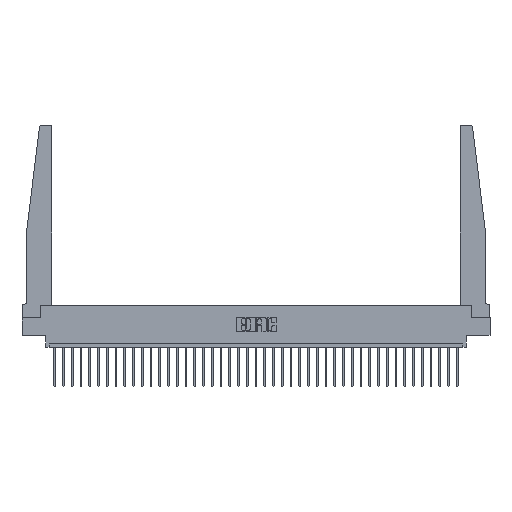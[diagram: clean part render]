
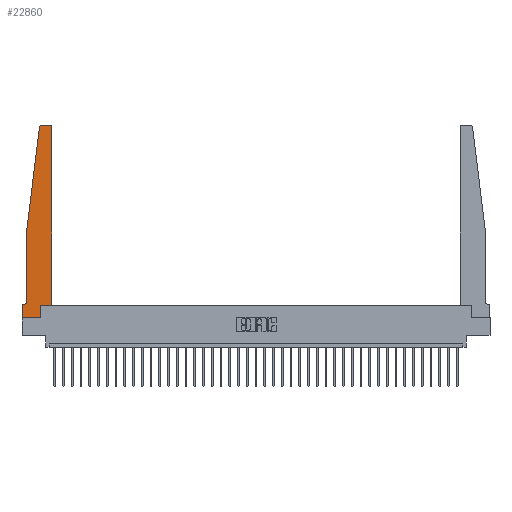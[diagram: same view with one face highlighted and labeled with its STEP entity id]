
A CAD part, top view. The second image highlights one B-rep face of the part: STEP entity #22860.
In plain terms, the highlighted planar face has unit normal (0, 0, 1).
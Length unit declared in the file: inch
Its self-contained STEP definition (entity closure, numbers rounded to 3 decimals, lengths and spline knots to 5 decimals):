
#249 = CARTESIAN_POINT ( 'NONE',  ( 0.065, 1.25, 0.37 ) ) ;
#384 = DIRECTION ( 'NONE',  ( 0., 1., 0. ) ) ;
#1217 = CIRCLE ( 'NONE', #8306, 0.03 ) ;
#1601 = CARTESIAN_POINT ( 'NONE',  ( 0.395, 2.75, 0.37 ) ) ;
#1854 = EDGE_CURVE ( 'NONE', #15519, #19445, #18045, .T. ) ;
#1911 = VECTOR ( 'NONE', #4742, 39.37008 ) ;
#2056 = AXIS2_PLACEMENT_3D ( 'NONE', #18401, #25612, #10159 ) ;
#2372 = CARTESIAN_POINT ( 'NONE',  ( 0.27653, 2.75, 0.37 ) ) ;
#3212 = LINE ( 'NONE', #31163, #17536 ) ;
#3720 = LINE ( 'NONE', #24644, #11105 ) ;
#3906 = VERTEX_POINT ( 'NONE', #32244 ) ;
#4670 = ORIENTED_EDGE ( 'NONE', *, *, #16605, .T. ) ;
#4693 = PLANE ( 'NONE',  #2056 ) ;
#4742 = DIRECTION ( 'NONE',  ( 1., 0., 0. ) ) ;
#4964 = CARTESIAN_POINT ( 'NONE',  ( 0.2605, 0.18, 0.37 ) ) ;
#5405 = ORIENTED_EDGE ( 'NONE', *, *, #1854, .T. ) ;
#6038 = EDGE_CURVE ( 'NONE', #16169, #17332, #11940, .T. ) ;
#6305 = EDGE_CURVE ( 'NONE', #3906, #33492, #29729, .T. ) ;
#7062 = CARTESIAN_POINT ( 'NONE',  ( 0., 0., 0.37 ) ) ;
#7340 = VECTOR ( 'NONE', #13923, 39.37008 ) ;
#7753 = CARTESIAN_POINT ( 'NONE',  ( 0., 0., 0.37 ) ) ;
#7915 = FACE_OUTER_BOUND ( 'NONE', #7938, .T. ) ;
#7938 = EDGE_LOOP ( 'NONE', ( #4670, #33658, #24033, #18374, #13474, #18819, #27400, #5405, #24749, #27364, #28347, #12217 ) ) ;
#8264 = DIRECTION ( 'NONE',  ( -1., 0., 0. ) ) ;
#8306 = AXIS2_PLACEMENT_3D ( 'NONE', #10468, #20936, #28463 ) ;
#8775 = LINE ( 'NONE', #10841, #7340 ) ;
#8815 = DIRECTION ( 'NONE',  ( 0., 0., 1. ) ) ;
#8956 = VECTOR ( 'NONE', #10697, 39.37008 ) ;
#9707 = LINE ( 'NONE', #25494, #1911 ) ;
#10068 = EDGE_CURVE ( 'NONE', #30839, #16169, #1217, .T. ) ;
#10159 = DIRECTION ( 'NONE',  ( 1., 0., 0. ) ) ;
#10468 = CARTESIAN_POINT ( 'NONE',  ( 0.27653, 2.72, 0.37 ) ) ;
#10549 = VECTOR ( 'NONE', #28042, 39.37008 ) ;
#10682 = LINE ( 'NONE', #18757, #19013 ) ;
#10697 = DIRECTION ( 'NONE',  ( -1., 0., 0. ) ) ;
#10841 = CARTESIAN_POINT ( 'NONE',  ( 0.2605, 0.18, 0.37 ) ) ;
#10946 = EDGE_CURVE ( 'NONE', #12994, #21836, #20360, .T. ) ;
#11105 = VECTOR ( 'NONE', #31818, 39.37008 ) ;
#11562 = CARTESIAN_POINT ( 'NONE',  ( 0.395, 2.72, 0.37 ) ) ;
#11940 = LINE ( 'NONE', #32853, #10549 ) ;
#12217 = ORIENTED_EDGE ( 'NONE', *, *, #6305, .T. ) ;
#12855 = CARTESIAN_POINT ( 'NONE',  ( 0.065, 0.2375, 0.37 ) ) ;
#12994 = VERTEX_POINT ( 'NONE', #12855 ) ;
#13065 = CARTESIAN_POINT ( 'NONE',  ( 0.425, 0.18, 0.37 ) ) ;
#13287 = AXIS2_PLACEMENT_3D ( 'NONE', #11562, #8815, #29732 ) ;
#13474 = ORIENTED_EDGE ( 'NONE', *, *, #10946, .T. ) ;
#13923 = DIRECTION ( 'NONE',  ( 0., 1., 0. ) ) ;
#15147 = EDGE_CURVE ( 'NONE', #21836, #23645, #17765, .T. ) ;
#15519 = VERTEX_POINT ( 'NONE', #7753 ) ;
#16169 = VERTEX_POINT ( 'NONE', #20392 ) ;
#16605 = EDGE_CURVE ( 'NONE', #33492, #30839, #3720, .T. ) ;
#16638 = CARTESIAN_POINT ( 'NONE',  ( 0.015, 0.1875, 0.37 ) ) ;
#17256 = EDGE_CURVE ( 'NONE', #19445, #19138, #8775, .T. ) ;
#17332 = VERTEX_POINT ( 'NONE', #249 ) ;
#17536 = VECTOR ( 'NONE', #18169, 39.37008 ) ;
#17765 = LINE ( 'NONE', #25645, #8956 ) ;
#17890 = EDGE_CURVE ( 'NONE', #19138, #26549, #9707, .T. ) ;
#17979 = CARTESIAN_POINT ( 'NONE',  ( 0.2605, 0., 0.37 ) ) ;
#18045 = LINE ( 'NONE', #7062, #32635 ) ;
#18169 = DIRECTION ( 'NONE',  ( 0., -1., 0. ) ) ;
#18374 = ORIENTED_EDGE ( 'NONE', *, *, #28454, .T. ) ;
#18401 = CARTESIAN_POINT ( 'NONE',  ( 0., 0.1875, 0.37 ) ) ;
#18740 = CARTESIAN_POINT ( 'NONE',  ( 0., 0.1875, 0.37 ) ) ;
#18757 = CARTESIAN_POINT ( 'NONE',  ( 0.065, 1.25, 0.37 ) ) ;
#18819 = ORIENTED_EDGE ( 'NONE', *, *, #15147, .T. ) ;
#19013 = VECTOR ( 'NONE', #26121, 39.37008 ) ;
#19138 = VERTEX_POINT ( 'NONE', #4964 ) ;
#19416 = CARTESIAN_POINT ( 'NONE',  ( 0.015, 0.2375, 0.37 ) ) ;
#19445 = VERTEX_POINT ( 'NONE', #17979 ) ;
#20360 = CIRCLE ( 'NONE', #33470, 0.05 ) ;
#20392 = CARTESIAN_POINT ( 'NONE',  ( 0.24675, 2.72367, 0.37 ) ) ;
#20654 = CARTESIAN_POINT ( 'NONE',  ( 0.425, 0.18, 0.37 ) ) ;
#20936 = DIRECTION ( 'NONE',  ( 0., 0., 1. ) ) ;
#21836 = VERTEX_POINT ( 'NONE', #16638 ) ;
#22860 = ADVANCED_FACE ( 'NONE', ( #7915 ), #4693, .T. ) ;
#23645 = VERTEX_POINT ( 'NONE', #18740 ) ;
#24033 = ORIENTED_EDGE ( 'NONE', *, *, #6038, .T. ) ;
#24644 = CARTESIAN_POINT ( 'NONE',  ( 0.25, 2.75, 0.37 ) ) ;
#24749 = ORIENTED_EDGE ( 'NONE', *, *, #17256, .T. ) ;
#25494 = CARTESIAN_POINT ( 'NONE',  ( 0.425, 0.18, 0.37 ) ) ;
#25612 = DIRECTION ( 'NONE',  ( 0., 0., 1. ) ) ;
#25645 = CARTESIAN_POINT ( 'NONE',  ( 0.065, 0.1875, 0.37 ) ) ;
#26121 = DIRECTION ( 'NONE',  ( 0., -1., 0. ) ) ;
#26405 = LINE ( 'NONE', #13065, #26588 ) ;
#26549 = VERTEX_POINT ( 'NONE', #20654 ) ;
#26588 = VECTOR ( 'NONE', #384, 39.37008 ) ;
#27364 = ORIENTED_EDGE ( 'NONE', *, *, #17890, .T. ) ;
#27400 = ORIENTED_EDGE ( 'NONE', *, *, #33040, .T. ) ;
#28042 = DIRECTION ( 'NONE',  ( -0.122, -0.992, 0. ) ) ;
#28347 = ORIENTED_EDGE ( 'NONE', *, *, #28791, .T. ) ;
#28454 = EDGE_CURVE ( 'NONE', #17332, #12994, #10682, .T. ) ;
#28463 = DIRECTION ( 'NONE',  ( 1., 0., 0. ) ) ;
#28791 = EDGE_CURVE ( 'NONE', #26549, #3906, #26405, .T. ) ;
#29729 = CIRCLE ( 'NONE', #13287, 0.03 ) ;
#29732 = DIRECTION ( 'NONE',  ( 1., 0., 0. ) ) ;
#30839 = VERTEX_POINT ( 'NONE', #2372 ) ;
#31163 = CARTESIAN_POINT ( 'NONE',  ( 0., 0., 0.37 ) ) ;
#31745 = DIRECTION ( 'NONE',  ( 0., 0., -1. ) ) ;
#31818 = DIRECTION ( 'NONE',  ( -1., 0., 0. ) ) ;
#32244 = CARTESIAN_POINT ( 'NONE',  ( 0.425, 2.72, 0.37 ) ) ;
#32635 = VECTOR ( 'NONE', #32949, 39.37008 ) ;
#32853 = CARTESIAN_POINT ( 'NONE',  ( 0.065, 1.25, 0.37 ) ) ;
#32949 = DIRECTION ( 'NONE',  ( 1., 0., 0. ) ) ;
#33040 = EDGE_CURVE ( 'NONE', #23645, #15519, #3212, .T. ) ;
#33470 = AXIS2_PLACEMENT_3D ( 'NONE', #19416, #31745, #8264 ) ;
#33492 = VERTEX_POINT ( 'NONE', #1601 ) ;
#33658 = ORIENTED_EDGE ( 'NONE', *, *, #10068, .T. ) ;
